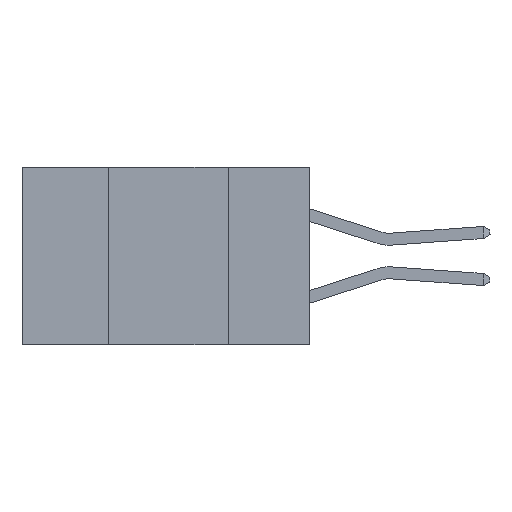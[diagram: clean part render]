
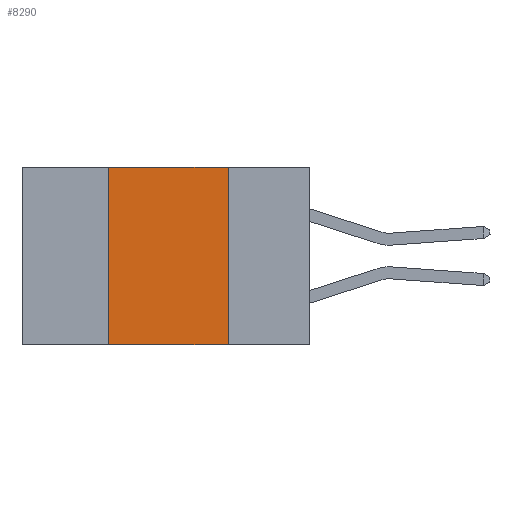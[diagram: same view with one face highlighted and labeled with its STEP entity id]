
A CAD part, left-side view. The second image highlights one B-rep face of the part: STEP entity #8290.
In plain terms, the highlighted planar face has unit normal (-1, 0, 0).
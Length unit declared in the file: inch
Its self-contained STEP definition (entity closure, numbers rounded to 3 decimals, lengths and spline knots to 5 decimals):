
#47 = CARTESIAN_POINT ( 'NONE',  ( 0., 0.17, -0.37 ) ) ;
#91 = DIRECTION ( 'NONE',  ( 0., -1., 0. ) ) ;
#1209 = VECTOR ( 'NONE', #91, 39.37008 ) ;
#1715 = ORIENTED_EDGE ( 'NONE', *, *, #3808, .F. ) ;
#2014 = CARTESIAN_POINT ( 'NONE',  ( 0., 0.17, -0.37 ) ) ;
#2154 = LINE ( 'NONE', #47, #5021 ) ;
#2244 = VERTEX_POINT ( 'NONE', #8577 ) ;
#2346 = LINE ( 'NONE', #13337, #1209 ) ;
#2670 = VERTEX_POINT ( 'NONE', #7635 ) ;
#3808 = EDGE_CURVE ( 'NONE', #2244, #9925, #2154, .T. ) ;
#3994 = VERTEX_POINT ( 'NONE', #4799 ) ;
#4041 = LINE ( 'NONE', #6184, #10174 ) ;
#4109 = EDGE_CURVE ( 'NONE', #2670, #3994, #4041, .T. ) ;
#4799 = CARTESIAN_POINT ( 'NONE',  ( 0., 0.42, 0. ) ) ;
#5021 = VECTOR ( 'NONE', #5234, 39.37008 ) ;
#5234 = DIRECTION ( 'NONE',  ( 0., 0., -1. ) ) ;
#5464 = FACE_OUTER_BOUND ( 'NONE', #13419, .T. ) ;
#6154 = ORIENTED_EDGE ( 'NONE', *, *, #9035, .F. ) ;
#6184 = CARTESIAN_POINT ( 'NONE',  ( 0., 0.42, -0.37 ) ) ;
#7635 = CARTESIAN_POINT ( 'NONE',  ( 0., 0.42, -0.37 ) ) ;
#8240 = ORIENTED_EDGE ( 'NONE', *, *, #14750, .T. ) ;
#8290 = ADVANCED_FACE ( 'NONE', ( #5464 ), #11987, .F. ) ;
#8577 = CARTESIAN_POINT ( 'NONE',  ( 0., 0.17, 0. ) ) ;
#9035 = EDGE_CURVE ( 'NONE', #3994, #2244, #13278, .T. ) ;
#9501 = DIRECTION ( 'NONE',  ( 0., -1., 0. ) ) ;
#9845 = VECTOR ( 'NONE', #9501, 39.37008 ) ;
#9925 = VERTEX_POINT ( 'NONE', #2014 ) ;
#10174 = VECTOR ( 'NONE', #13110, 39.37008 ) ;
#11646 = DIRECTION ( 'NONE',  ( 0., 0., -1. ) ) ;
#11751 = DIRECTION ( 'NONE',  ( 1., 0., 0. ) ) ;
#11951 = CARTESIAN_POINT ( 'NONE',  ( 0., 0.6, 0. ) ) ;
#11987 = PLANE ( 'NONE',  #12328 ) ;
#12073 = CARTESIAN_POINT ( 'NONE',  ( 0., 0.6, 0. ) ) ;
#12328 = AXIS2_PLACEMENT_3D ( 'NONE', #11951, #11751, #11646 ) ;
#13110 = DIRECTION ( 'NONE',  ( 0., 0., 1. ) ) ;
#13278 = LINE ( 'NONE', #12073, #9845 ) ;
#13337 = CARTESIAN_POINT ( 'NONE',  ( 0., 0.6, -0.37 ) ) ;
#13419 = EDGE_LOOP ( 'NONE', ( #1715, #6154, #13906, #8240 ) ) ;
#13906 = ORIENTED_EDGE ( 'NONE', *, *, #4109, .F. ) ;
#14750 = EDGE_CURVE ( 'NONE', #2670, #9925, #2346, .T. ) ;
